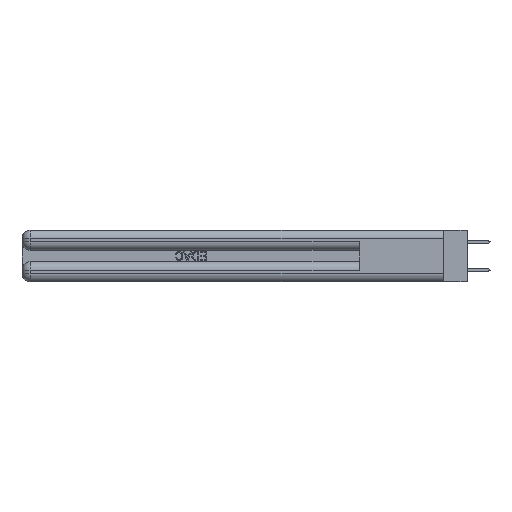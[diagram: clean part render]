
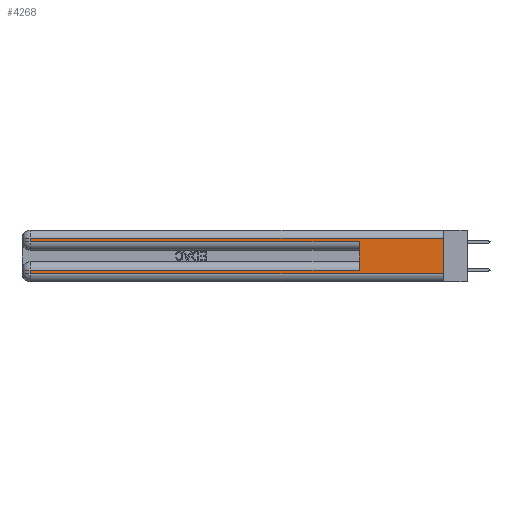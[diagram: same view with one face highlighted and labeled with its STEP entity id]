
A CAD part, left-side view. The second image highlights one B-rep face of the part: STEP entity #4268.
In plain terms, the highlighted planar face has unit normal (-1, 0, 0).
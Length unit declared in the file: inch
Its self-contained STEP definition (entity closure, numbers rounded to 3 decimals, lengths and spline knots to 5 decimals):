
#823 = CARTESIAN_POINT ( 'NONE',  ( 0., 2.94, 0.085 ) ) ;
#1402 = DIRECTION ( 'NONE',  ( 0., 1., 0. ) ) ;
#1808 = ORIENTED_EDGE ( 'NONE', *, *, #28816, .T. ) ;
#1822 = CARTESIAN_POINT ( 'NONE',  ( 0., 0., 0.37 ) ) ;
#2155 = FACE_OUTER_BOUND ( 'NONE', #2825, .T. ) ;
#2283 = ORIENTED_EDGE ( 'NONE', *, *, #4871, .F. ) ;
#2588 = LINE ( 'NONE', #7926, #9941 ) ;
#2825 = EDGE_LOOP ( 'NONE', ( #2283, #18934, #37354, #32095, #8186, #34021, #1808, #35922 ) ) ;
#4268 = ADVANCED_FACE ( 'NONE', ( #2155 ), #39083, .F. ) ;
#4282 = EDGE_CURVE ( 'NONE', #16642, #9467, #17834, .T. ) ;
#4871 = EDGE_CURVE ( 'NONE', #28720, #7117, #2588, .T. ) ;
#5232 = CARTESIAN_POINT ( 'NONE',  ( 0., 0., 0.285 ) ) ;
#6067 = LINE ( 'NONE', #24249, #29012 ) ;
#6857 = EDGE_CURVE ( 'NONE', #11357, #7071, #30761, .T. ) ;
#7071 = VERTEX_POINT ( 'NONE', #30729 ) ;
#7117 = VERTEX_POINT ( 'NONE', #33969 ) ;
#7926 = CARTESIAN_POINT ( 'NONE',  ( 0., 0., 0.37 ) ) ;
#8039 = LINE ( 'NONE', #5232, #23708 ) ;
#8131 = DIRECTION ( 'NONE',  ( 0., 0., -1. ) ) ;
#8186 = ORIENTED_EDGE ( 'NONE', *, *, #4282, .F. ) ;
#8384 = DIRECTION ( 'NONE',  ( 0., -1., 0. ) ) ;
#9467 = VERTEX_POINT ( 'NONE', #32621 ) ;
#9629 = VECTOR ( 'NONE', #38986, 39.37008 ) ;
#9941 = VECTOR ( 'NONE', #35951, 39.37008 ) ;
#11357 = VERTEX_POINT ( 'NONE', #34548 ) ;
#13128 = CARTESIAN_POINT ( 'NONE',  ( 0., 0.6, 0.085 ) ) ;
#13384 = AXIS2_PLACEMENT_3D ( 'NONE', #1822, #26829, #8131 ) ;
#14973 = DIRECTION ( 'NONE',  ( 0., 1., 0. ) ) ;
#16642 = VERTEX_POINT ( 'NONE', #13128 ) ;
#16904 = CARTESIAN_POINT ( 'NONE',  ( 0., 0., 0.085 ) ) ;
#17322 = CARTESIAN_POINT ( 'NONE',  ( 0., 2.94, 0.37 ) ) ;
#17834 = LINE ( 'NONE', #33077, #24193 ) ;
#17924 = DIRECTION ( 'NONE',  ( 0., -1., 0. ) ) ;
#18934 = ORIENTED_EDGE ( 'NONE', *, *, #23816, .T. ) ;
#19672 = VERTEX_POINT ( 'NONE', #823 ) ;
#20684 = DIRECTION ( 'NONE',  ( 0., 0., 1. ) ) ;
#22492 = VECTOR ( 'NONE', #23035, 39.37008 ) ;
#23035 = DIRECTION ( 'NONE',  ( 0., 0., -1. ) ) ;
#23700 = EDGE_CURVE ( 'NONE', #7071, #9467, #8039, .T. ) ;
#23708 = VECTOR ( 'NONE', #8384, 39.37008 ) ;
#23816 = EDGE_CURVE ( 'NONE', #28720, #11357, #6067, .T. ) ;
#23992 = EDGE_CURVE ( 'NONE', #36021, #7117, #33390, .T. ) ;
#24193 = VECTOR ( 'NONE', #20684, 39.37008 ) ;
#24249 = CARTESIAN_POINT ( 'NONE',  ( 0., 0., 0.31 ) ) ;
#24291 = LINE ( 'NONE', #17322, #9629 ) ;
#26829 = DIRECTION ( 'NONE',  ( 1., 0., 0. ) ) ;
#27332 = VECTOR ( 'NONE', #1402, 39.37008 ) ;
#27459 = EDGE_CURVE ( 'NONE', #16642, #19672, #35531, .T. ) ;
#28720 = VERTEX_POINT ( 'NONE', #29294 ) ;
#28816 = EDGE_CURVE ( 'NONE', #19672, #36021, #24291, .T. ) ;
#29012 = VECTOR ( 'NONE', #14973, 39.37008 ) ;
#29294 = CARTESIAN_POINT ( 'NONE',  ( 0., 0., 0.31 ) ) ;
#30729 = CARTESIAN_POINT ( 'NONE',  ( 0., 2.94, 0.285 ) ) ;
#30761 = LINE ( 'NONE', #32253, #22492 ) ;
#32095 = ORIENTED_EDGE ( 'NONE', *, *, #23700, .T. ) ;
#32253 = CARTESIAN_POINT ( 'NONE',  ( 0., 2.94, 0.37 ) ) ;
#32321 = CARTESIAN_POINT ( 'NONE',  ( 0., 2.94, 0.06 ) ) ;
#32621 = CARTESIAN_POINT ( 'NONE',  ( 0., 0.6, 0.285 ) ) ;
#33077 = CARTESIAN_POINT ( 'NONE',  ( 0., 0.6, 0.145 ) ) ;
#33390 = LINE ( 'NONE', #37310, #39580 ) ;
#33969 = CARTESIAN_POINT ( 'NONE',  ( 0., 0., 0.06 ) ) ;
#34021 = ORIENTED_EDGE ( 'NONE', *, *, #27459, .T. ) ;
#34548 = CARTESIAN_POINT ( 'NONE',  ( 0., 2.94, 0.31 ) ) ;
#35531 = LINE ( 'NONE', #16904, #27332 ) ;
#35922 = ORIENTED_EDGE ( 'NONE', *, *, #23992, .T. ) ;
#35951 = DIRECTION ( 'NONE',  ( 0., 0., -1. ) ) ;
#36021 = VERTEX_POINT ( 'NONE', #32321 ) ;
#37310 = CARTESIAN_POINT ( 'NONE',  ( 0., 0., 0.06 ) ) ;
#37354 = ORIENTED_EDGE ( 'NONE', *, *, #6857, .T. ) ;
#38986 = DIRECTION ( 'NONE',  ( 0., 0., -1. ) ) ;
#39083 = PLANE ( 'NONE',  #13384 ) ;
#39580 = VECTOR ( 'NONE', #17924, 39.37008 ) ;
